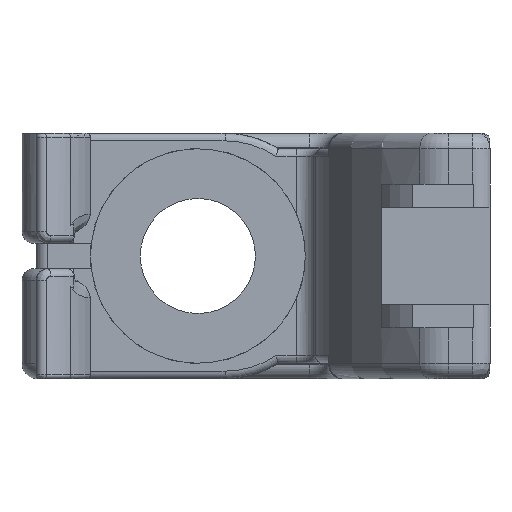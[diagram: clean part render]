
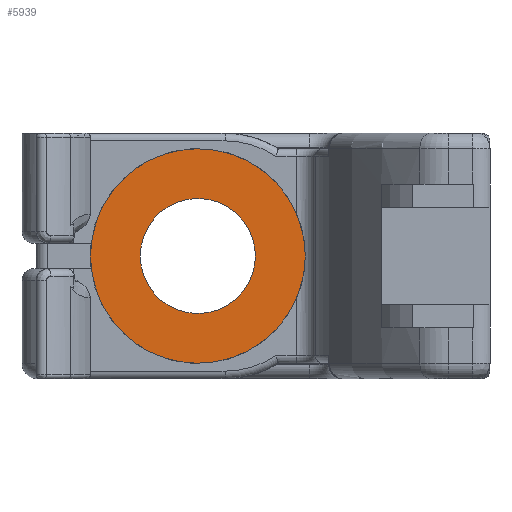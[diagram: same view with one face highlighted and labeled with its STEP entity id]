
A CAD part, left-side view. The second image highlights one B-rep face of the part: STEP entity #5939.
In plain terms, the highlighted planar face has unit normal (-1, 0, 0).
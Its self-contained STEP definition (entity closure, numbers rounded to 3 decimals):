
#152=FACE_BOUND('',#2084,.T.);
#226=PLANE('',#6371);
#1734=FACE_OUTER_BOUND('',#2083,.T.);
#2083=EDGE_LOOP('',(#4603));
#2084=EDGE_LOOP('',(#4604));
#2377=CIRCLE('',#6276,14.);
#2402=CIRCLE('',#6372,7.5);
#2672=VERTEX_POINT('',#8803);
#2848=VERTEX_POINT('',#9438);
#3259=EDGE_CURVE('',#2672,#2672,#2377,.T.);
#3505=EDGE_CURVE('',#2848,#2848,#2402,.T.);
#4603=ORIENTED_EDGE('',*,*,#3259,.F.);
#4604=ORIENTED_EDGE('',*,*,#3505,.T.);
#5939=ADVANCED_FACE('',(#1734,#152),#226,.F.);
#6276=AXIS2_PLACEMENT_3D('',#8805,#6969,#6970);
#6371=AXIS2_PLACEMENT_3D('',#9437,#7357,#7358);
#6372=AXIS2_PLACEMENT_3D('',#9439,#7359,#7360);
#6969=DIRECTION('center_axis',(1.,0.,0.));
#6970=DIRECTION('ref_axis',(0.,-1.,0.));
#7357=DIRECTION('center_axis',(1.,0.,0.));
#7358=DIRECTION('ref_axis',(0.,1.,0.));
#7359=DIRECTION('center_axis',(1.,0.,0.));
#7360=DIRECTION('ref_axis',(0.,-1.,0.));
#8803=CARTESIAN_POINT('',(0.38,13.126,3.664));
#8805=CARTESIAN_POINT('Origin',(0.38,-0.874,3.664));
#9437=CARTESIAN_POINT('Origin',(0.38,-12.91,3.664));
#9438=CARTESIAN_POINT('',(0.38,6.626,3.664));
#9439=CARTESIAN_POINT('Origin',(0.38,-0.874,3.664));
